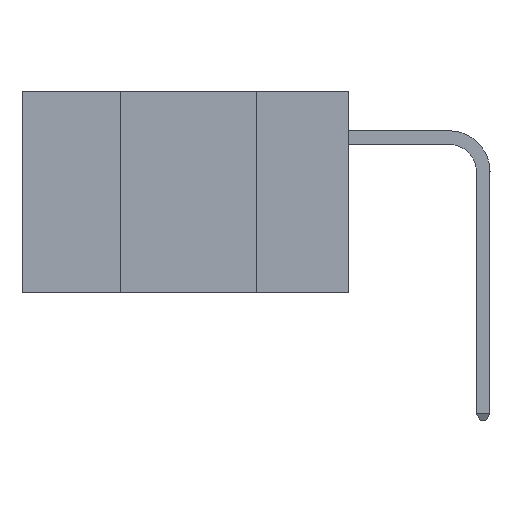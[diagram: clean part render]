
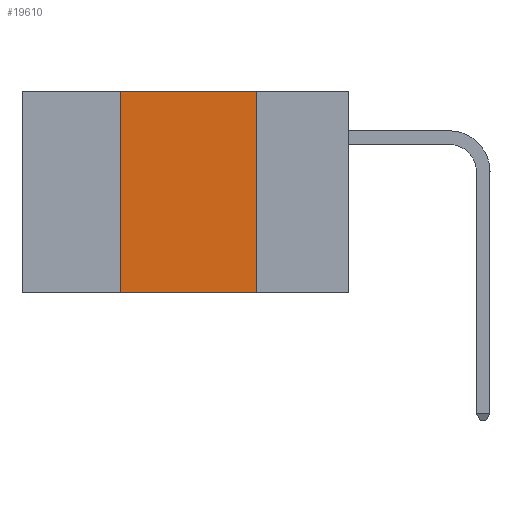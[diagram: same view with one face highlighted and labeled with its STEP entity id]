
A CAD part, left-side view. The second image highlights one B-rep face of the part: STEP entity #19610.
In plain terms, the highlighted planar face has unit normal (-1, 0, 0).
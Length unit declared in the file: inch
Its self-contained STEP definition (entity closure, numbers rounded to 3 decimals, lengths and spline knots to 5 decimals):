
#421 = CARTESIAN_POINT ( 'NONE',  ( 0., 0.42, 0. ) ) ;
#655 = EDGE_CURVE ( 'NONE', #12012, #10502, #12270, .T. ) ;
#1142 = LINE ( 'NONE', #12986, #18022 ) ;
#1345 = CARTESIAN_POINT ( 'NONE',  ( 0., 0.42, 0. ) ) ;
#3444 = PLANE ( 'NONE',  #11953 ) ;
#6187 = DIRECTION ( 'NONE',  ( 0., -1., 0. ) ) ;
#6473 = EDGE_CURVE ( 'NONE', #12229, #20833, #1142, .T. ) ;
#7014 = ORIENTED_EDGE ( 'NONE', *, *, #22442, .F. ) ;
#7784 = EDGE_LOOP ( 'NONE', ( #15941, #7014, #16072, #15522 ) ) ;
#9003 = CARTESIAN_POINT ( 'NONE',  ( 0., 0.17, 0. ) ) ;
#10293 = LINE ( 'NONE', #24334, #23702 ) ;
#10409 = FACE_OUTER_BOUND ( 'NONE', #7784, .T. ) ;
#10502 = VERTEX_POINT ( 'NONE', #1345 ) ;
#11552 = DIRECTION ( 'NONE',  ( 1., 0., 0. ) ) ;
#11856 = DIRECTION ( 'NONE',  ( 0., -1., 0. ) ) ;
#11953 = AXIS2_PLACEMENT_3D ( 'NONE', #13490, #11552, #15037 ) ;
#12012 = VERTEX_POINT ( 'NONE', #18276 ) ;
#12229 = VERTEX_POINT ( 'NONE', #9003 ) ;
#12270 = LINE ( 'NONE', #421, #14924 ) ;
#12595 = DIRECTION ( 'NONE',  ( 0., 0., -1. ) ) ;
#12986 = CARTESIAN_POINT ( 'NONE',  ( 0., 0.17, 0. ) ) ;
#13227 = EDGE_CURVE ( 'NONE', #12012, #20833, #13297, .T. ) ;
#13297 = LINE ( 'NONE', #19469, #24923 ) ;
#13490 = CARTESIAN_POINT ( 'NONE',  ( 0., 0.6, 0. ) ) ;
#14924 = VECTOR ( 'NONE', #22323, 39.37008 ) ;
#15037 = DIRECTION ( 'NONE',  ( 0., 0., -1. ) ) ;
#15522 = ORIENTED_EDGE ( 'NONE', *, *, #13227, .T. ) ;
#15941 = ORIENTED_EDGE ( 'NONE', *, *, #6473, .F. ) ;
#16072 = ORIENTED_EDGE ( 'NONE', *, *, #655, .F. ) ;
#18022 = VECTOR ( 'NONE', #12595, 39.37008 ) ;
#18276 = CARTESIAN_POINT ( 'NONE',  ( 0., 0.42, -0.37 ) ) ;
#18782 = CARTESIAN_POINT ( 'NONE',  ( 0., 0.17, -0.37 ) ) ;
#19469 = CARTESIAN_POINT ( 'NONE',  ( 0., 0.6, -0.37 ) ) ;
#19610 = ADVANCED_FACE ( 'NONE', ( #10409 ), #3444, .F. ) ;
#20833 = VERTEX_POINT ( 'NONE', #18782 ) ;
#22323 = DIRECTION ( 'NONE',  ( 0., 0., 1. ) ) ;
#22442 = EDGE_CURVE ( 'NONE', #10502, #12229, #10293, .T. ) ;
#23702 = VECTOR ( 'NONE', #6187, 39.37008 ) ;
#24334 = CARTESIAN_POINT ( 'NONE',  ( 0., 0.6, 0. ) ) ;
#24923 = VECTOR ( 'NONE', #11856, 39.37008 ) ;
